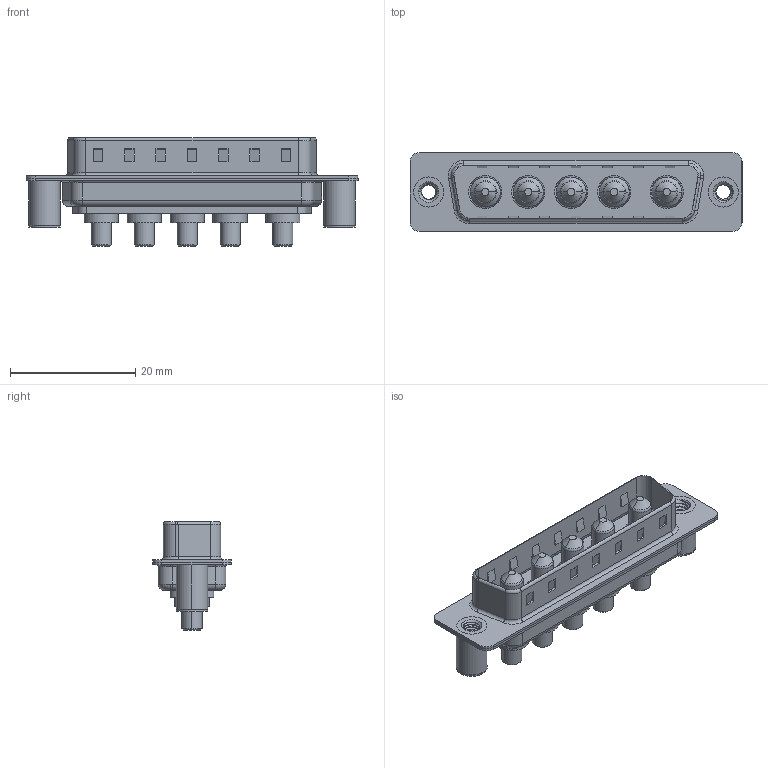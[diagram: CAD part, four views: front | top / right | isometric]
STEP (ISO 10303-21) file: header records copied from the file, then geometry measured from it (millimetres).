
FILE_DESCRIPTION (( 'STEP AP203' ), '1' );
FILE_NAME ('627-5W5-224-3NB.STEP', '2019-05-25T20:32:02', ( '' ), ( '' ), 'SwSTEP 2.0', 'SolidWorks 2016', '' );
FILE_SCHEMA (( 'CONFIG_CONTROL_DESIGN' ));
Length unit declared in the file: millimetre
Products named in the file (7): 627Combo Shell Front_25 Contacts; 627Combo Threaded Board Spacer_B; 627Combo Housing_5W5; Power Pin_30A S; 627Combo Shell Rear_25 Contacts; 627Combo Threaded Board Spacer_3; 627-5W5-224-3NB
Assembly tree (10 placements, depth 2):
  627-5W5-224-3NB
    627Combo Housing_5W5
    627Combo Shell Rear_25 Contacts
    627Combo Shell Front_25 Contacts
    627Combo Threaded Board Spacer_B
    Power Pin_30A S  x5
    627Combo Threaded Board Spacer_3
Bounding box: 53 x 12.6 x 17.4 mm (x, y, z)
Volume: 3222.7 mm3; surface area: 6949.5 mm2
Topology: 15 solids, 15 shells, 614 faces, 1477 edges, 919 vertices
Faces by surface type: cylinder 260, plane 221, torus 64, cone 53, bspline 16
Entity records: 18518 total; most frequent: CARTESIAN_POINT 6262, DIRECTION 2440, ORIENTED_EDGE 2366, EDGE_CURVE 1183, AXIS2_PLACEMENT_3D 900, VERTEX_POINT 743, VECTOR 640, LINE 640
